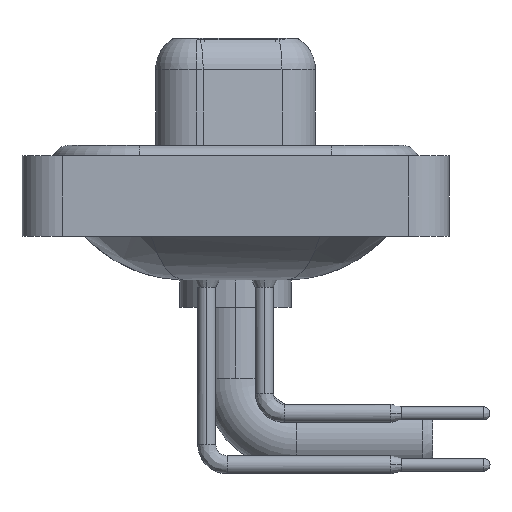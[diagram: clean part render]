
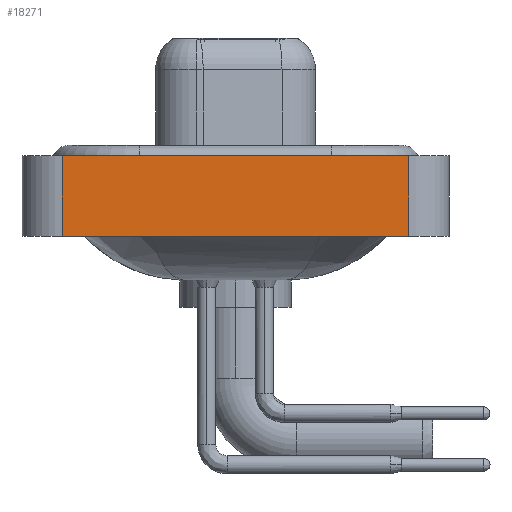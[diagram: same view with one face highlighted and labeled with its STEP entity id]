
A CAD part, left-side view. The second image highlights one B-rep face of the part: STEP entity #18271.
In plain terms, the highlighted planar face has unit normal (-1, 0, 0).
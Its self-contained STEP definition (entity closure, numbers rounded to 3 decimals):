
#215 = EDGE_LOOP ( 'NONE', ( #826, #2910, #17472, #15604 ) ) ;
#826 = ORIENTED_EDGE ( 'NONE', *, *, #3111, .T. ) ;
#950 = FACE_OUTER_BOUND ( 'NONE', #215, .T. ) ;
#1409 = CARTESIAN_POINT ( 'NONE',  ( -7.25, -8.55, 0.4 ) ) ;
#1503 = AXIS2_PLACEMENT_3D ( 'NONE', #19371, #13270, #16564 ) ;
#1581 = EDGE_CURVE ( 'NONE', #13662, #18880, #17996, .T. ) ;
#2696 = CARTESIAN_POINT ( 'NONE',  ( -7.25, 8.55, -3.6 ) ) ;
#2838 = PLANE ( 'NONE',  #1503 ) ;
#2910 = ORIENTED_EDGE ( 'NONE', *, *, #1581, .F. ) ;
#3111 = EDGE_CURVE ( 'NONE', #13002, #18880, #13471, .T. ) ;
#3552 = CARTESIAN_POINT ( 'NONE',  ( -7.25, -8.55, -3.6 ) ) ;
#4552 = DIRECTION ( 'NONE',  ( 0., 0., 1. ) ) ;
#5613 = DIRECTION ( 'NONE',  ( 0., 0., 1. ) ) ;
#8161 = DIRECTION ( 'NONE',  ( 0., -1., 0. ) ) ;
#8722 = LINE ( 'NONE', #2696, #14117 ) ;
#9687 = CARTESIAN_POINT ( 'NONE',  ( -7.25, -8.55, -3.6 ) ) ;
#10455 = EDGE_CURVE ( 'NONE', #15181, #13662, #8722, .T. ) ;
#12178 = VECTOR ( 'NONE', #13490, 1000. ) ;
#12897 = VECTOR ( 'NONE', #4552, 1000. ) ;
#13002 = VERTEX_POINT ( 'NONE', #3552 ) ;
#13270 = DIRECTION ( 'NONE',  ( -1., 0., 0. ) ) ;
#13471 = LINE ( 'NONE', #19565, #12897 ) ;
#13490 = DIRECTION ( 'NONE',  ( 0., -1., 0. ) ) ;
#13627 = CARTESIAN_POINT ( 'NONE',  ( -7.25, 8.55, -3.6 ) ) ;
#13662 = VERTEX_POINT ( 'NONE', #16142 ) ;
#14117 = VECTOR ( 'NONE', #5613, 1000. ) ;
#15181 = VERTEX_POINT ( 'NONE', #13627 ) ;
#15604 = ORIENTED_EDGE ( 'NONE', *, *, #16187, .T. ) ;
#16142 = CARTESIAN_POINT ( 'NONE',  ( -7.25, 8.55, 0.4 ) ) ;
#16187 = EDGE_CURVE ( 'NONE', #15181, #13002, #19344, .T. ) ;
#16564 = DIRECTION ( 'NONE',  ( 0., 0., 1. ) ) ;
#17472 = ORIENTED_EDGE ( 'NONE', *, *, #10455, .F. ) ;
#17893 = CARTESIAN_POINT ( 'NONE',  ( -7.25, -8.55, 0.4 ) ) ;
#17996 = LINE ( 'NONE', #17893, #12178 ) ;
#18271 = ADVANCED_FACE ( 'NONE', ( #950 ), #2838, .T. ) ;
#18880 = VERTEX_POINT ( 'NONE', #1409 ) ;
#19344 = LINE ( 'NONE', #9687, #19722 ) ;
#19371 = CARTESIAN_POINT ( 'NONE',  ( -7.25, -8.55, -3.6 ) ) ;
#19565 = CARTESIAN_POINT ( 'NONE',  ( -7.25, -8.55, -3.6 ) ) ;
#19722 = VECTOR ( 'NONE', #8161, 1000. ) ;
